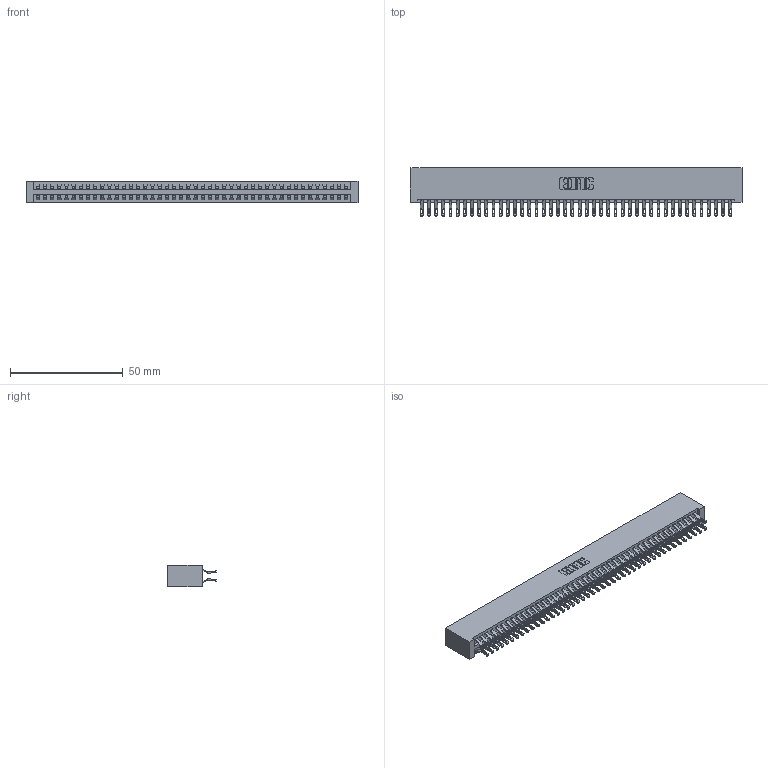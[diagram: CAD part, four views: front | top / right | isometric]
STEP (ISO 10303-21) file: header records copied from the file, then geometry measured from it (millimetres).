
FILE_DESCRIPTION (( 'STEP AP203' ), '1' );
FILE_NAME ('396-088-555-201.STEP', '2019-10-31T01:26:01', ( '' ), ( '' ), 'SwSTEP 2.0', 'SolidWorks 2016', '' );
FILE_SCHEMA (( 'CONFIG_CONTROL_DESIGN' ));
Length unit declared in the file: inch
Products named in the file (3): 346 Part_No Mounting Lugs; 396-088-555-201; 345-292-001_555 Tail
Assembly tree (89 placements, depth 2):
  396-088-555-201
    346 Part_No Mounting Lugs
    345-292-001_555 Tail  x88
Bounding box: 146.94 x 21.46 x 9.4 mm (x, y, z)
Volume: 15172.4 mm3; surface area: 21960 mm2
Topology: 89 solids, 89 shells, 5218 faces, 16409 edges, 10938 vertices
Faces by surface type: plane 2976, cylinder 2242
Entity records: 28495 total; most frequent: CARTESIAN_POINT 4726, ORIENTED_EDGE 4630, DIRECTION 4179, EDGE_CURVE 2315, VECTOR 1995, LINE 1995, VERTEX_POINT 1542, AXIS2_PLACEMENT_3D 1092
